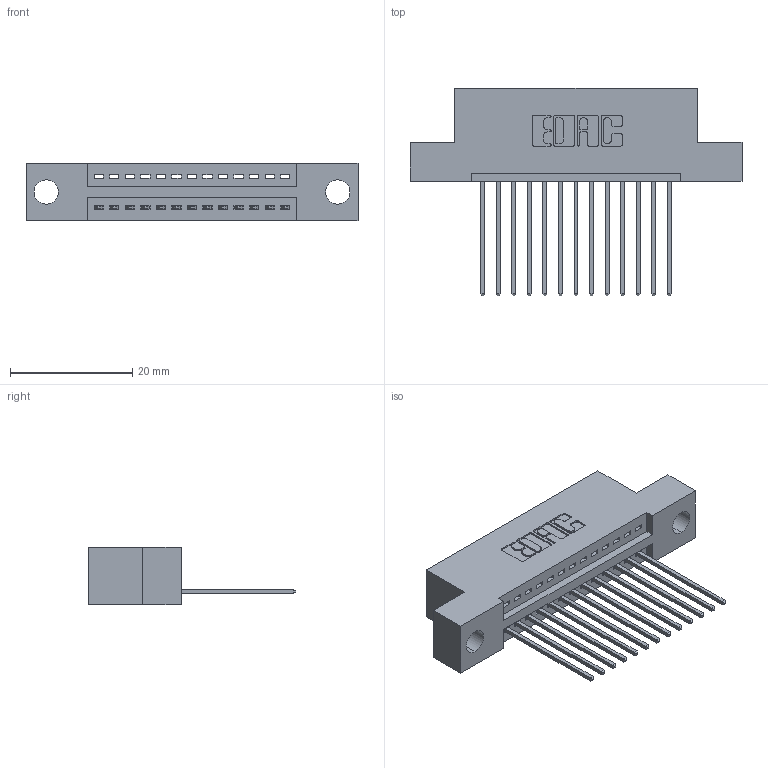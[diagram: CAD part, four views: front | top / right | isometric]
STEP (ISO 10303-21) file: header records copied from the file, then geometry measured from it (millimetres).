
FILE_DESCRIPTION (( 'STEP AP203' ), '1' );
FILE_NAME ('395-013-541-104.STEP', '2021-05-31T14:19:15', ( '' ), ( '' ), 'SwSTEP 2.0', 'SolidWorks 2020', '' );
FILE_SCHEMA (( 'CONFIG_CONTROL_DESIGN' ));
Length unit declared in the file: inch
Products named in the file (3): 345-292-001_345-293-141; 345 Part_Flush Mounting Lugs - 0.156 Dia-TI; 395-013-541-104
Assembly tree (14 placements, depth 2):
  395-013-541-104
    345 Part_Flush Mounting Lugs - 0.156 Dia-TI
    345-292-001_345-293-141  x13
Bounding box: 54.23 x 33.96 x 9.4 mm (x, y, z)
Volume: 4850.1 mm3; surface area: 6146.1 mm2
Topology: 14 solids, 14 shells, 894 faces, 2665 edges, 1758 vertices
Faces by surface type: plane 614, cylinder 280
Entity records: 14125 total; most frequent: CARTESIAN_POINT 2457, ORIENTED_EDGE 2402, DIRECTION 2187, EDGE_CURVE 1201, VECTOR 1017, LINE 1017, VERTEX_POINT 798, AXIS2_PLACEMENT_3D 585
